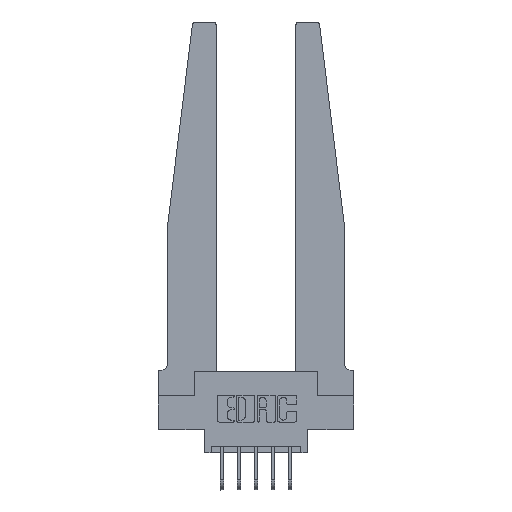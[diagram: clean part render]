
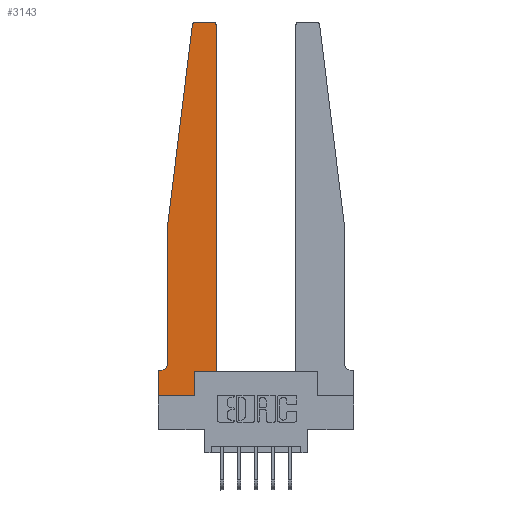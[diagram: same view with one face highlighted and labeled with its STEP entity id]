
A CAD part, top view. The second image highlights one B-rep face of the part: STEP entity #3143.
In plain terms, the highlighted planar face has unit normal (0, 0, 1).
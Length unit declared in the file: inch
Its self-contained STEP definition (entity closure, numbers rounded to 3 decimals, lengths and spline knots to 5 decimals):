
#77 = DIRECTION ( 'NONE',  ( 0., 0., 1. ) ) ;
#282 = CARTESIAN_POINT ( 'NONE',  ( 0.425, 0.18, 0.37 ) ) ;
#298 = CARTESIAN_POINT ( 'NONE',  ( 0.015, 0.2375, 0.37 ) ) ;
#394 = DIRECTION ( 'NONE',  ( 0., 0., -1. ) ) ;
#668 = EDGE_CURVE ( 'NONE', #11603, #9311, #4534, .T. ) ;
#672 = CARTESIAN_POINT ( 'NONE',  ( 0.25, 2.75, 0.37 ) ) ;
#742 = DIRECTION ( 'NONE',  ( 0., -1., 0. ) ) ;
#827 = EDGE_CURVE ( 'NONE', #13563, #5570, #8495, .T. ) ;
#906 = LINE ( 'NONE', #5232, #6656 ) ;
#1116 = CARTESIAN_POINT ( 'NONE',  ( 0.2605, 0.18, 0.37 ) ) ;
#1185 = PLANE ( 'NONE',  #7469 ) ;
#1250 = CARTESIAN_POINT ( 'NONE',  ( 0.065, 1.25, 0.37 ) ) ;
#1454 = DIRECTION ( 'NONE',  ( -1., 0., 0. ) ) ;
#1589 = EDGE_CURVE ( 'NONE', #9311, #5352, #5155, .T. ) ;
#1963 = VERTEX_POINT ( 'NONE', #3605 ) ;
#2157 = FACE_OUTER_BOUND ( 'NONE', #9341, .T. ) ;
#2318 = DIRECTION ( 'NONE',  ( 0., 0., 1. ) ) ;
#2334 = DIRECTION ( 'NONE',  ( 0., -1., 0. ) ) ;
#2681 = VECTOR ( 'NONE', #8580, 39.37008 ) ;
#2926 = VERTEX_POINT ( 'NONE', #9636 ) ;
#3143 = ADVANCED_FACE ( 'NONE', ( #2157 ), #1185, .T. ) ;
#3463 = CARTESIAN_POINT ( 'NONE',  ( 0.27653, 2.72, 0.37 ) ) ;
#3577 = CARTESIAN_POINT ( 'NONE',  ( 0.015, 0.1875, 0.37 ) ) ;
#3605 = CARTESIAN_POINT ( 'NONE',  ( 0.2605, 0., 0.37 ) ) ;
#4439 = CARTESIAN_POINT ( 'NONE',  ( 0.395, 2.75, 0.37 ) ) ;
#4534 = LINE ( 'NONE', #1250, #7797 ) ;
#4661 = DIRECTION ( 'NONE',  ( 1., 0., 0. ) ) ;
#5007 = VECTOR ( 'NONE', #742, 39.37008 ) ;
#5041 = EDGE_CURVE ( 'NONE', #5570, #8493, #12295, .T. ) ;
#5155 = CIRCLE ( 'NONE', #6475, 0.05 ) ;
#5232 = CARTESIAN_POINT ( 'NONE',  ( 0.065, 0.1875, 0.37 ) ) ;
#5352 = VERTEX_POINT ( 'NONE', #3577 ) ;
#5370 = CARTESIAN_POINT ( 'NONE',  ( 0.425, 0.18, 0.37 ) ) ;
#5491 = ORIENTED_EDGE ( 'NONE', *, *, #8644, .T. ) ;
#5549 = DIRECTION ( 'NONE',  ( 0., 1., 0. ) ) ;
#5570 = VERTEX_POINT ( 'NONE', #4439 ) ;
#5790 = VERTEX_POINT ( 'NONE', #9518 ) ;
#5824 = CARTESIAN_POINT ( 'NONE',  ( 0., 0.1875, 0.37 ) ) ;
#6280 = ORIENTED_EDGE ( 'NONE', *, *, #7173, .T. ) ;
#6375 = ORIENTED_EDGE ( 'NONE', *, *, #10920, .T. ) ;
#6420 = DIRECTION ( 'NONE',  ( -1., 0., 0. ) ) ;
#6475 = AXIS2_PLACEMENT_3D ( 'NONE', #298, #394, #1454 ) ;
#6490 = LINE ( 'NONE', #282, #11511 ) ;
#6597 = LINE ( 'NONE', #5370, #8415 ) ;
#6656 = VECTOR ( 'NONE', #6420, 39.37008 ) ;
#6929 = VECTOR ( 'NONE', #5549, 39.37008 ) ;
#7093 = DIRECTION ( 'NONE',  ( 0., 0., 1. ) ) ;
#7112 = EDGE_CURVE ( 'NONE', #8973, #11521, #6597, .T. ) ;
#7173 = EDGE_CURVE ( 'NONE', #1963, #8973, #9839, .T. ) ;
#7380 = CARTESIAN_POINT ( 'NONE',  ( 0.425, 0.18, 0.37 ) ) ;
#7469 = AXIS2_PLACEMENT_3D ( 'NONE', #5824, #2318, #4661 ) ;
#7663 = LINE ( 'NONE', #12581, #14362 ) ;
#7797 = VECTOR ( 'NONE', #2334, 39.37008 ) ;
#7799 = ORIENTED_EDGE ( 'NONE', *, *, #13929, .T. ) ;
#8133 = CIRCLE ( 'NONE', #8849, 0.03 ) ;
#8142 = DIRECTION ( 'NONE',  ( 1., 0., 0. ) ) ;
#8325 = DIRECTION ( 'NONE',  ( 1., 0., 0. ) ) ;
#8415 = VECTOR ( 'NONE', #10010, 39.37008 ) ;
#8493 = VERTEX_POINT ( 'NONE', #11611 ) ;
#8495 = CIRCLE ( 'NONE', #13035, 0.03 ) ;
#8580 = DIRECTION ( 'NONE',  ( -1., 0., 0. ) ) ;
#8644 = EDGE_CURVE ( 'NONE', #5352, #2926, #906, .T. ) ;
#8647 = CARTESIAN_POINT ( 'NONE',  ( 0., 0., 0.37 ) ) ;
#8674 = ORIENTED_EDGE ( 'NONE', *, *, #5041, .T. ) ;
#8849 = AXIS2_PLACEMENT_3D ( 'NONE', #3463, #77, #12566 ) ;
#8973 = VERTEX_POINT ( 'NONE', #1116 ) ;
#9311 = VERTEX_POINT ( 'NONE', #13575 ) ;
#9328 = VERTEX_POINT ( 'NONE', #8647 ) ;
#9341 = EDGE_LOOP ( 'NONE', ( #8674, #7799, #13464, #14893, #10012, #5491, #6375, #12747, #6280, #9937, #14683, #9810 ) ) ;
#9518 = CARTESIAN_POINT ( 'NONE',  ( 0.24675, 2.72367, 0.37 ) ) ;
#9636 = CARTESIAN_POINT ( 'NONE',  ( 0., 0.1875, 0.37 ) ) ;
#9810 = ORIENTED_EDGE ( 'NONE', *, *, #827, .T. ) ;
#9839 = LINE ( 'NONE', #13572, #6929 ) ;
#9937 = ORIENTED_EDGE ( 'NONE', *, *, #7112, .T. ) ;
#10010 = DIRECTION ( 'NONE',  ( 1., 0., 0. ) ) ;
#10012 = ORIENTED_EDGE ( 'NONE', *, *, #1589, .T. ) ;
#10584 = CARTESIAN_POINT ( 'NONE',  ( 0.065, 1.25, 0.37 ) ) ;
#10668 = CARTESIAN_POINT ( 'NONE',  ( 0.395, 2.72, 0.37 ) ) ;
#10683 = VECTOR ( 'NONE', #12890, 39.37008 ) ;
#10920 = EDGE_CURVE ( 'NONE', #2926, #9328, #12956, .T. ) ;
#10989 = CARTESIAN_POINT ( 'NONE',  ( 0., 0., 0.37 ) ) ;
#11511 = VECTOR ( 'NONE', #12998, 39.37008 ) ;
#11521 = VERTEX_POINT ( 'NONE', #7380 ) ;
#11574 = LINE ( 'NONE', #14604, #10683 ) ;
#11603 = VERTEX_POINT ( 'NONE', #10584 ) ;
#11611 = CARTESIAN_POINT ( 'NONE',  ( 0.27653, 2.75, 0.37 ) ) ;
#12203 = EDGE_CURVE ( 'NONE', #11521, #13563, #6490, .T. ) ;
#12295 = LINE ( 'NONE', #672, #2681 ) ;
#12518 = CARTESIAN_POINT ( 'NONE',  ( 0.425, 2.72, 0.37 ) ) ;
#12566 = DIRECTION ( 'NONE',  ( 1., 0., 0. ) ) ;
#12581 = CARTESIAN_POINT ( 'NONE',  ( 0., 0., 0.37 ) ) ;
#12747 = ORIENTED_EDGE ( 'NONE', *, *, #13060, .T. ) ;
#12890 = DIRECTION ( 'NONE',  ( -0.122, -0.992, 0. ) ) ;
#12956 = LINE ( 'NONE', #10989, #5007 ) ;
#12998 = DIRECTION ( 'NONE',  ( 0., 1., 0. ) ) ;
#13035 = AXIS2_PLACEMENT_3D ( 'NONE', #10668, #7093, #8325 ) ;
#13060 = EDGE_CURVE ( 'NONE', #9328, #1963, #7663, .T. ) ;
#13464 = ORIENTED_EDGE ( 'NONE', *, *, #14827, .T. ) ;
#13563 = VERTEX_POINT ( 'NONE', #12518 ) ;
#13572 = CARTESIAN_POINT ( 'NONE',  ( 0.2605, 0.18, 0.37 ) ) ;
#13575 = CARTESIAN_POINT ( 'NONE',  ( 0.065, 0.2375, 0.37 ) ) ;
#13929 = EDGE_CURVE ( 'NONE', #8493, #5790, #8133, .T. ) ;
#14362 = VECTOR ( 'NONE', #8142, 39.37008 ) ;
#14604 = CARTESIAN_POINT ( 'NONE',  ( 0.065, 1.25, 0.37 ) ) ;
#14683 = ORIENTED_EDGE ( 'NONE', *, *, #12203, .T. ) ;
#14827 = EDGE_CURVE ( 'NONE', #5790, #11603, #11574, .T. ) ;
#14893 = ORIENTED_EDGE ( 'NONE', *, *, #668, .T. ) ;
